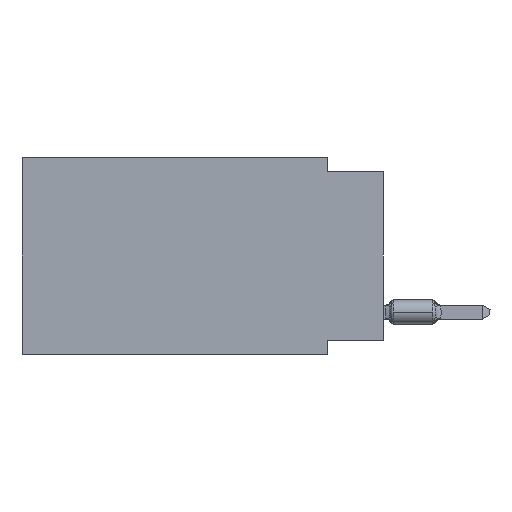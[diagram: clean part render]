
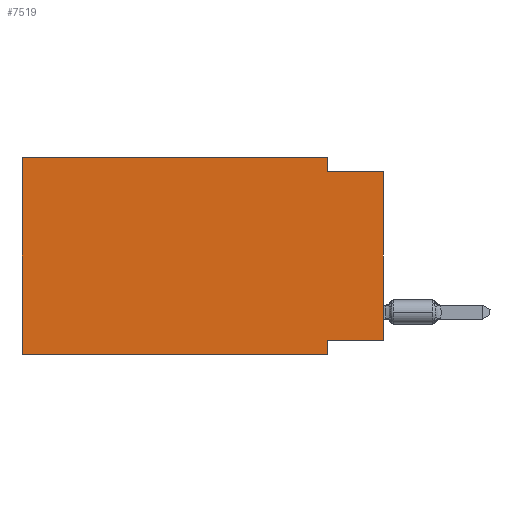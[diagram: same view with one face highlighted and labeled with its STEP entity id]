
A CAD part, left-side view. The second image highlights one B-rep face of the part: STEP entity #7519.
In plain terms, the highlighted planar face has unit normal (-1, 0, 0).
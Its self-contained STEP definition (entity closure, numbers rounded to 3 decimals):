
#241 = LINE ( 'NONE', #31329, #10495 ) ;
#624 = VERTEX_POINT ( 'NONE', #21681 ) ;
#3211 = LINE ( 'NONE', #26492, #25204 ) ;
#3869 = VERTEX_POINT ( 'NONE', #31480 ) ;
#4495 = DIRECTION ( 'NONE',  ( 0., 1., 0. ) ) ;
#4720 = ORIENTED_EDGE ( 'NONE', *, *, #22607, .F. ) ;
#5270 = DIRECTION ( 'NONE',  ( 0., -1., 0. ) ) ;
#5617 = VERTEX_POINT ( 'NONE', #6744 ) ;
#6671 = LINE ( 'NONE', #29621, #33161 ) ;
#6744 = CARTESIAN_POINT ( 'NONE',  ( 0., 0., -0.635 ) ) ;
#7202 = LINE ( 'NONE', #25252, #19730 ) ;
#7519 = ADVANCED_FACE ( 'NONE', ( #12860 ), #22710, .F. ) ;
#7960 = EDGE_LOOP ( 'NONE', ( #9500, #32870, #33576, #30094, #4720, #27963, #15923, #23398 ) ) ;
#9500 = ORIENTED_EDGE ( 'NONE', *, *, #23908, .T. ) ;
#9769 = DIRECTION ( 'NONE',  ( 0., 0., -1. ) ) ;
#9946 = DIRECTION ( 'NONE',  ( 1., 0., 0. ) ) ;
#10347 = LINE ( 'NONE', #28699, #33292 ) ;
#10495 = VECTOR ( 'NONE', #10761, 1000. ) ;
#10761 = DIRECTION ( 'NONE',  ( 0., -1., 0. ) ) ;
#10795 = CARTESIAN_POINT ( 'NONE',  ( 0., 0., -8.255 ) ) ;
#11782 = VERTEX_POINT ( 'NONE', #22329 ) ;
#12860 = FACE_OUTER_BOUND ( 'NONE', #7960, .T. ) ;
#12999 = EDGE_CURVE ( 'NONE', #31414, #3869, #16045, .T. ) ;
#13583 = DIRECTION ( 'NONE',  ( 0., -1., 0. ) ) ;
#13964 = DIRECTION ( 'NONE',  ( 0., 0., 1. ) ) ;
#14033 = CARTESIAN_POINT ( 'NONE',  ( 0., 16.383, 0. ) ) ;
#15075 = CARTESIAN_POINT ( 'NONE',  ( 0., 16.383, 0. ) ) ;
#15192 = VECTOR ( 'NONE', #28269, 1000. ) ;
#15923 = ORIENTED_EDGE ( 'NONE', *, *, #22450, .F. ) ;
#16045 = LINE ( 'NONE', #25919, #15192 ) ;
#17593 = VERTEX_POINT ( 'NONE', #14033 ) ;
#19730 = VECTOR ( 'NONE', #4495, 1000. ) ;
#20336 = AXIS2_PLACEMENT_3D ( 'NONE', #15075, #9946, #9769 ) ;
#20354 = VECTOR ( 'NONE', #13964, 1000. ) ;
#20378 = VERTEX_POINT ( 'NONE', #10795 ) ;
#20712 = EDGE_CURVE ( 'NONE', #20378, #33144, #7202, .T. ) ;
#20863 = EDGE_CURVE ( 'NONE', #11782, #624, #241, .T. ) ;
#21681 = CARTESIAN_POINT ( 'NONE',  ( 0., 2.54, -8.89 ) ) ;
#21768 = EDGE_CURVE ( 'NONE', #17593, #31414, #3211, .T. ) ;
#22329 = CARTESIAN_POINT ( 'NONE',  ( 0., 16.383, -8.89 ) ) ;
#22450 = EDGE_CURVE ( 'NONE', #33144, #624, #26373, .T. ) ;
#22607 = EDGE_CURVE ( 'NONE', #11782, #17593, #32117, .T. ) ;
#22710 = PLANE ( 'NONE',  #20336 ) ;
#22907 = CARTESIAN_POINT ( 'NONE',  ( 0., 2.54, -8.255 ) ) ;
#23398 = ORIENTED_EDGE ( 'NONE', *, *, #20712, .F. ) ;
#23819 = DIRECTION ( 'NONE',  ( 0., 0., -1. ) ) ;
#23908 = EDGE_CURVE ( 'NONE', #20378, #5617, #6671, .T. ) ;
#24681 = VECTOR ( 'NONE', #23819, 1000. ) ;
#25204 = VECTOR ( 'NONE', #13583, 1000. ) ;
#25252 = CARTESIAN_POINT ( 'NONE',  ( 0., 0., -8.255 ) ) ;
#25919 = CARTESIAN_POINT ( 'NONE',  ( 0., 2.54, 0. ) ) ;
#26037 = CARTESIAN_POINT ( 'NONE',  ( 0., 2.54, -8.89 ) ) ;
#26373 = LINE ( 'NONE', #26037, #24681 ) ;
#26492 = CARTESIAN_POINT ( 'NONE',  ( 0., 16.383, 0. ) ) ;
#27963 = ORIENTED_EDGE ( 'NONE', *, *, #20863, .T. ) ;
#28269 = DIRECTION ( 'NONE',  ( 0., 0., -1. ) ) ;
#28699 = CARTESIAN_POINT ( 'NONE',  ( 0., 0., -0.635 ) ) ;
#29621 = CARTESIAN_POINT ( 'NONE',  ( 0., 0., 0. ) ) ;
#30094 = ORIENTED_EDGE ( 'NONE', *, *, #21768, .F. ) ;
#31329 = CARTESIAN_POINT ( 'NONE',  ( 0., 16.383, -8.89 ) ) ;
#31414 = VERTEX_POINT ( 'NONE', #32229 ) ;
#31480 = CARTESIAN_POINT ( 'NONE',  ( 0., 2.54, -0.635 ) ) ;
#32117 = LINE ( 'NONE', #32455, #20354 ) ;
#32229 = CARTESIAN_POINT ( 'NONE',  ( 0., 2.54, 0. ) ) ;
#32339 = DIRECTION ( 'NONE',  ( 0., 0., 1. ) ) ;
#32455 = CARTESIAN_POINT ( 'NONE',  ( 0., 16.383, 0. ) ) ;
#32797 = EDGE_CURVE ( 'NONE', #3869, #5617, #10347, .T. ) ;
#32870 = ORIENTED_EDGE ( 'NONE', *, *, #32797, .F. ) ;
#33144 = VERTEX_POINT ( 'NONE', #22907 ) ;
#33161 = VECTOR ( 'NONE', #32339, 1000. ) ;
#33292 = VECTOR ( 'NONE', #5270, 1000. ) ;
#33576 = ORIENTED_EDGE ( 'NONE', *, *, #12999, .F. ) ;
